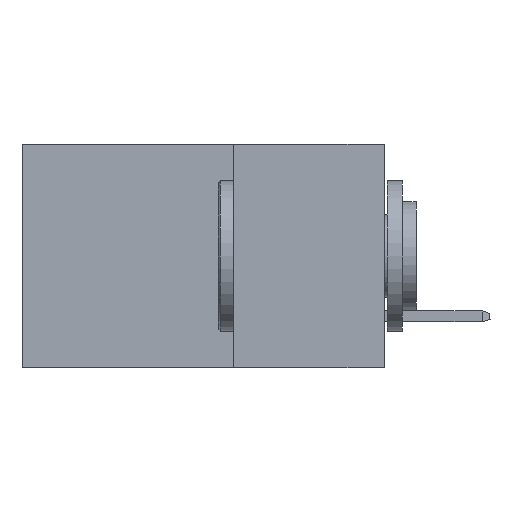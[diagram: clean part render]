
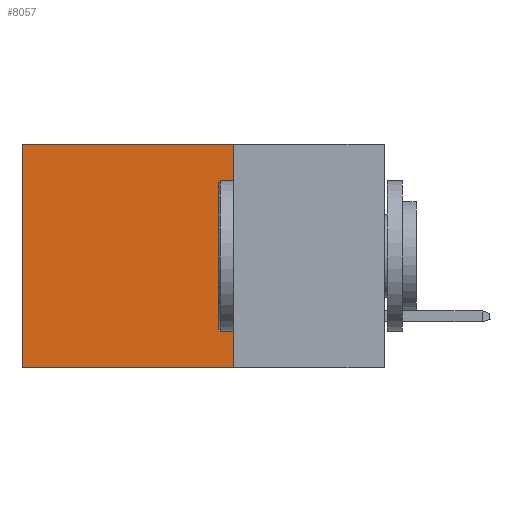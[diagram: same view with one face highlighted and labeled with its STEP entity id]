
A CAD part, left-side view. The second image highlights one B-rep face of the part: STEP entity #8057.
In plain terms, the highlighted planar face has unit normal (-1, 0, 0).
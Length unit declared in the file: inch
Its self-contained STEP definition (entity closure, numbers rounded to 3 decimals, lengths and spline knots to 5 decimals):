
#342 = VERTEX_POINT ( 'NONE', #4169 ) ;
#1086 = ORIENTED_EDGE ( 'NONE', *, *, #8629, .F. ) ;
#1376 = FACE_OUTER_BOUND ( 'NONE', #10025, .T. ) ;
#1609 = CARTESIAN_POINT ( 'NONE',  ( 0.2615, 0.6, -0.37 ) ) ;
#1685 = EDGE_CURVE ( 'NONE', #12176, #7219, #6012, .T. ) ;
#1912 = DIRECTION ( 'NONE',  ( 1., 0., 0. ) ) ;
#2049 = PLANE ( 'NONE',  #6800 ) ;
#2500 = ORIENTED_EDGE ( 'NONE', *, *, #1685, .F. ) ;
#2533 = VERTEX_POINT ( 'NONE', #3081 ) ;
#3081 = CARTESIAN_POINT ( 'NONE',  ( 0.2615, 0.25, 0. ) ) ;
#4133 = DIRECTION ( 'NONE',  ( 0., 0., -1. ) ) ;
#4169 = CARTESIAN_POINT ( 'NONE',  ( 0.2615, 0.6, 0. ) ) ;
#4604 = VECTOR ( 'NONE', #13001, 39.37008 ) ;
#5212 = CARTESIAN_POINT ( 'NONE',  ( 0.2615, 0.25, 0. ) ) ;
#5353 = DIRECTION ( 'NONE',  ( 0., 0., -1. ) ) ;
#5720 = CARTESIAN_POINT ( 'NONE',  ( 0.2615, 0.25, -0.37 ) ) ;
#6012 = LINE ( 'NONE', #5720, #9346 ) ;
#6165 = ORIENTED_EDGE ( 'NONE', *, *, #10252, .T. ) ;
#6730 = EDGE_CURVE ( 'NONE', #2533, #342, #7234, .T. ) ;
#6800 = AXIS2_PLACEMENT_3D ( 'NONE', #10906, #1912, #5353 ) ;
#7219 = VERTEX_POINT ( 'NONE', #1609 ) ;
#7234 = LINE ( 'NONE', #5212, #4604 ) ;
#7501 = DIRECTION ( 'NONE',  ( 0., 0., -1. ) ) ;
#7810 = DIRECTION ( 'NONE',  ( 0., 1., 0. ) ) ;
#8032 = VECTOR ( 'NONE', #7501, 39.37008 ) ;
#8057 = ADVANCED_FACE ( 'NONE', ( #1376 ), #2049, .F. ) ;
#8629 = EDGE_CURVE ( 'NONE', #2533, #12176, #11014, .T. ) ;
#8908 = ORIENTED_EDGE ( 'NONE', *, *, #6730, .T. ) ;
#8944 = CARTESIAN_POINT ( 'NONE',  ( 0.2615, 0.25, -0.37 ) ) ;
#9346 = VECTOR ( 'NONE', #7810, 39.37008 ) ;
#10025 = EDGE_LOOP ( 'NONE', ( #6165, #2500, #1086, #8908 ) ) ;
#10252 = EDGE_CURVE ( 'NONE', #342, #7219, #10968, .T. ) ;
#10795 = CARTESIAN_POINT ( 'NONE',  ( 0.2615, 0.25, -0.37 ) ) ;
#10906 = CARTESIAN_POINT ( 'NONE',  ( 0.2615, 0.25, -0.37 ) ) ;
#10968 = LINE ( 'NONE', #11551, #8032 ) ;
#11014 = LINE ( 'NONE', #10795, #11371 ) ;
#11371 = VECTOR ( 'NONE', #4133, 39.37008 ) ;
#11551 = CARTESIAN_POINT ( 'NONE',  ( 0.2615, 0.6, -0.37 ) ) ;
#12176 = VERTEX_POINT ( 'NONE', #8944 ) ;
#13001 = DIRECTION ( 'NONE',  ( 0., 1., 0. ) ) ;
